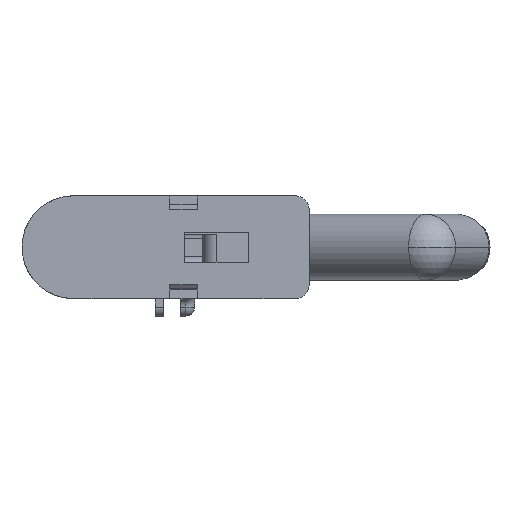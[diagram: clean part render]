
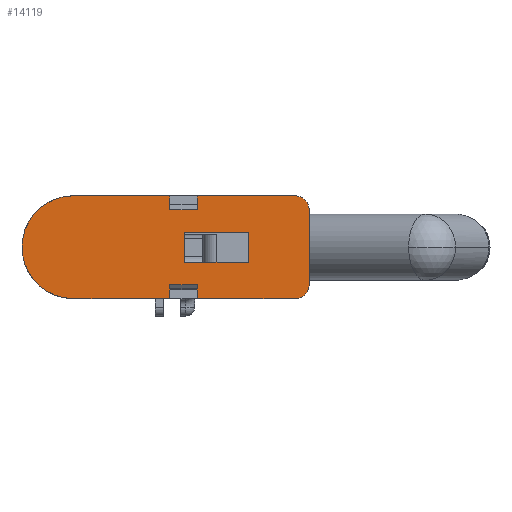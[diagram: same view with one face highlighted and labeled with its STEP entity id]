
A CAD part, left-side view. The second image highlights one B-rep face of the part: STEP entity #14119.
In plain terms, the highlighted planar face has unit normal (-1, 0, 0).
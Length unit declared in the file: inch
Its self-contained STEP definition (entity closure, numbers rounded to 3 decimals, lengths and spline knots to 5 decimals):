
#7 = EDGE_CURVE ( 'NONE', #6480, #2978, #19024, .T. ) ;
#82 = EDGE_CURVE ( 'NONE', #23408, #14286, #2425, .T. ) ;
#172 = DIRECTION ( 'NONE',  ( 0., -1., 0. ) ) ;
#319 = CARTESIAN_POINT ( 'NONE',  ( -5.00064, -0.77841, -0.73097 ) ) ;
#370 = DIRECTION ( 'NONE',  ( -1., 0., 0. ) ) ;
#374 = CARTESIAN_POINT ( 'NONE',  ( -5.00064, -1.89702, 0.21654 ) ) ;
#472 = VERTEX_POINT ( 'NONE', #2930 ) ;
#625 = EDGE_CURVE ( 'NONE', #23710, #17356, #10900, .T. ) ;
#834 = CARTESIAN_POINT ( 'NONE',  ( -5.00064, -0.47716, -0.73097 ) ) ;
#877 = CARTESIAN_POINT ( 'NONE',  ( -5.00064, -2.76317, -0.73097 ) ) ;
#1217 = DIRECTION ( 'NONE',  ( 0., -1., 0. ) ) ;
#1369 = CARTESIAN_POINT ( 'NONE',  ( -5.00064, -1.17211, 0.53412 ) ) ;
#1397 = AXIS2_PLACEMENT_3D ( 'NONE', #12386, #370, #14398 ) ;
#2003 = VECTOR ( 'NONE', #4301, 39.37008 ) ;
#2425 = LINE ( 'NONE', #16116, #3072 ) ;
#2536 = CARTESIAN_POINT ( 'NONE',  ( -5.00064, 0.59382, 0. ) ) ;
#2633 = PLANE ( 'NONE',  #14245 ) ;
#2685 = EDGE_CURVE ( 'NONE', #14286, #5938, #12403, .T. ) ;
#2930 = CARTESIAN_POINT ( 'NONE',  ( -5.00064, -0.77841, -0.53412 ) ) ;
#2978 = VERTEX_POINT ( 'NONE', #20927 ) ;
#3072 = VECTOR ( 'NONE', #172, 39.37008 ) ;
#3211 = ORIENTED_EDGE ( 'NONE', *, *, #15143, .F. ) ;
#3433 = VECTOR ( 'NONE', #15560, 39.37008 ) ;
#3440 = VECTOR ( 'NONE', #15381, 39.37008 ) ;
#3620 = CARTESIAN_POINT ( 'NONE',  ( -5.00064, 0.6158, -0.73097 ) ) ;
#3667 = VECTOR ( 'NONE', #13679, 39.37008 ) ;
#3846 = LINE ( 'NONE', #23876, #19196 ) ;
#3899 = VECTOR ( 'NONE', #14204, 39.37008 ) ;
#4105 = VERTEX_POINT ( 'NONE', #319 ) ;
#4142 = CARTESIAN_POINT ( 'NONE',  ( -5.00064, -0.77841, 0.73097 ) ) ;
#4150 = LINE ( 'NONE', #7176, #24799 ) ;
#4214 = ORIENTED_EDGE ( 'NONE', *, *, #7452, .F. ) ;
#4301 = DIRECTION ( 'NONE',  ( 0., 0., 1. ) ) ;
#4498 = ORIENTED_EDGE ( 'NONE', *, *, #82, .F. ) ;
#4556 = DIRECTION ( 'NONE',  ( 0., 0., 1. ) ) ;
#4612 = ORIENTED_EDGE ( 'NONE', *, *, #17510, .F. ) ;
#4621 = CARTESIAN_POINT ( 'NONE',  ( -5.00064, 0.6158, 0.73097 ) ) ;
#5158 = LINE ( 'NONE', #19234, #25776 ) ;
#5443 = CARTESIAN_POINT ( 'NONE',  ( -5.00064, -1.89702, -0.21654 ) ) ;
#5496 = CARTESIAN_POINT ( 'NONE',  ( -5.00064, -0.77841, -0.73097 ) ) ;
#5601 = AXIS2_PLACEMENT_3D ( 'NONE', #2536, #16521, #4556 ) ;
#5738 = ORIENTED_EDGE ( 'NONE', *, *, #7, .F. ) ;
#5938 = VERTEX_POINT ( 'NONE', #374 ) ;
#6448 = ORIENTED_EDGE ( 'NONE', *, *, #7729, .F. ) ;
#6480 = VERTEX_POINT ( 'NONE', #14417 ) ;
#6512 = DIRECTION ( 'NONE',  ( 0., -1., 0. ) ) ;
#6532 = VECTOR ( 'NONE', #23488, 39.37008 ) ;
#6745 = CARTESIAN_POINT ( 'NONE',  ( -5.00064, 2.30886, -16.99949 ) ) ;
#6814 = EDGE_CURVE ( 'NONE', #11249, #6480, #18746, .T. ) ;
#7101 = VECTOR ( 'NONE', #22167, 39.37008 ) ;
#7171 = CARTESIAN_POINT ( 'NONE',  ( -5.00064, -2.56632, 0.53412 ) ) ;
#7176 = CARTESIAN_POINT ( 'NONE',  ( -5.00064, -0.47716, 0.73097 ) ) ;
#7179 = LINE ( 'NONE', #5496, #6532 ) ;
#7230 = CARTESIAN_POINT ( 'NONE',  ( -5.00064, -0.99151, 0.21654 ) ) ;
#7359 = LINE ( 'NONE', #12258, #2003 ) ;
#7452 = EDGE_CURVE ( 'NONE', #18812, #13443, #23778, .T. ) ;
#7729 = EDGE_CURVE ( 'NONE', #2978, #19135, #8129, .T. ) ;
#7967 = CIRCLE ( 'NONE', #1397, 0.19685 ) ;
#8129 = LINE ( 'NONE', #1369, #3440 ) ;
#8660 = ORIENTED_EDGE ( 'NONE', *, *, #18913, .F. ) ;
#9104 = EDGE_LOOP ( 'NONE', ( #6448, #5738, #21211, #20274, #4214, #25468, #23220, #15988, #4612, #10188, #17609, #23754, #13958, #8660 ) ) ;
#9213 = DIRECTION ( 'NONE',  ( 0., 0., 1. ) ) ;
#9797 = CARTESIAN_POINT ( 'NONE',  ( -5.00064, -0.77841, 0.73097 ) ) ;
#9852 = CARTESIAN_POINT ( 'NONE',  ( -5.00064, -0.77841, 0.53412 ) ) ;
#10070 = VECTOR ( 'NONE', #6512, 39.37008 ) ;
#10188 = ORIENTED_EDGE ( 'NONE', *, *, #15830, .T. ) ;
#10584 = CARTESIAN_POINT ( 'NONE',  ( -5.00064, -1.17211, -0.73097 ) ) ;
#10761 = VERTEX_POINT ( 'NONE', #7230 ) ;
#10817 = EDGE_LOOP ( 'NONE', ( #3211, #17130, #4498, #11124 ) ) ;
#10900 = CIRCLE ( 'NONE', #15709, 0.19685 ) ;
#11124 = ORIENTED_EDGE ( 'NONE', *, *, #17986, .T. ) ;
#11249 = VERTEX_POINT ( 'NONE', #4142 ) ;
#11300 = CARTESIAN_POINT ( 'NONE',  ( -5.00064, -2.76317, 0.53412 ) ) ;
#12134 = EDGE_CURVE ( 'NONE', #14852, #472, #13526, .T. ) ;
#12141 = FACE_OUTER_BOUND ( 'NONE', #9104, .T. ) ;
#12258 = CARTESIAN_POINT ( 'NONE',  ( -5.00064, -1.17211, -0.73097 ) ) ;
#12386 = CARTESIAN_POINT ( 'NONE',  ( -5.00064, -2.56632, -0.53412 ) ) ;
#12403 = LINE ( 'NONE', #24191, #7101 ) ;
#12825 = DIRECTION ( 'NONE',  ( 0., -1., 0. ) ) ;
#13294 = DIRECTION ( 'NONE',  ( 0., 0., 1. ) ) ;
#13336 = DIRECTION ( 'NONE',  ( 0., 1., 0. ) ) ;
#13443 = VERTEX_POINT ( 'NONE', #4621 ) ;
#13526 = LINE ( 'NONE', #25294, #23520 ) ;
#13679 = DIRECTION ( 'NONE',  ( 0., 1., 0. ) ) ;
#13720 = VECTOR ( 'NONE', #21796, 39.37008 ) ;
#13932 = DIRECTION ( 'NONE',  ( 0., -1., 0. ) ) ;
#13958 = ORIENTED_EDGE ( 'NONE', *, *, #625, .T. ) ;
#14119 = ADVANCED_FACE ( 'NONE', ( #12141, #17473 ), #2633, .T. ) ;
#14204 = DIRECTION ( 'NONE',  ( 0., 0., 1. ) ) ;
#14245 = AXIS2_PLACEMENT_3D ( 'NONE', #6745, #16624, #22737 ) ;
#14286 = VERTEX_POINT ( 'NONE', #5443 ) ;
#14312 = LINE ( 'NONE', #23639, #3667 ) ;
#14398 = DIRECTION ( 'NONE',  ( 0., 0., 1. ) ) ;
#14417 = CARTESIAN_POINT ( 'NONE',  ( -5.00064, -0.77841, 0.53412 ) ) ;
#14553 = LINE ( 'NONE', #877, #3899 ) ;
#14852 = VERTEX_POINT ( 'NONE', #24321 ) ;
#15143 = EDGE_CURVE ( 'NONE', #5938, #10761, #14312, .T. ) ;
#15381 = DIRECTION ( 'NONE',  ( 0., 0., 1. ) ) ;
#15401 = LINE ( 'NONE', #20504, #10070 ) ;
#15560 = DIRECTION ( 'NONE',  ( 0., 0., -1. ) ) ;
#15709 = AXIS2_PLACEMENT_3D ( 'NONE', #7171, #21174, #9213 ) ;
#15830 = EDGE_CURVE ( 'NONE', #16779, #16683, #23048, .T. ) ;
#15988 = ORIENTED_EDGE ( 'NONE', *, *, #12134, .F. ) ;
#16116 = CARTESIAN_POINT ( 'NONE',  ( -5.00064, 0., -0.21654 ) ) ;
#16521 = DIRECTION ( 'NONE',  ( 1., 0., 0. ) ) ;
#16623 = CARTESIAN_POINT ( 'NONE',  ( -5.00064, -2.76317, -0.53412 ) ) ;
#16624 = DIRECTION ( 'NONE',  ( -1., 0., 0. ) ) ;
#16683 = VERTEX_POINT ( 'NONE', #18884 ) ;
#16779 = VERTEX_POINT ( 'NONE', #10584 ) ;
#17130 = ORIENTED_EDGE ( 'NONE', *, *, #2685, .F. ) ;
#17356 = VERTEX_POINT ( 'NONE', #19100 ) ;
#17473 = FACE_BOUND ( 'NONE', #10817, .T. ) ;
#17510 = EDGE_CURVE ( 'NONE', #16779, #14852, #7359, .T. ) ;
#17609 = ORIENTED_EDGE ( 'NONE', *, *, #18152, .T. ) ;
#17986 = EDGE_CURVE ( 'NONE', #23408, #10761, #5158, .T. ) ;
#18152 = EDGE_CURVE ( 'NONE', #16683, #19073, #7967, .T. ) ;
#18746 = LINE ( 'NONE', #9797, #3433 ) ;
#18812 = VERTEX_POINT ( 'NONE', #3620 ) ;
#18884 = CARTESIAN_POINT ( 'NONE',  ( -5.00064, -2.56632, -0.73097 ) ) ;
#18913 = EDGE_CURVE ( 'NONE', #19135, #17356, #3846, .T. ) ;
#19024 = LINE ( 'NONE', #9852, #13720 ) ;
#19073 = VERTEX_POINT ( 'NONE', #16623 ) ;
#19100 = CARTESIAN_POINT ( 'NONE',  ( -5.00064, -2.56632, 0.73097 ) ) ;
#19135 = VERTEX_POINT ( 'NONE', #22823 ) ;
#19196 = VECTOR ( 'NONE', #13932, 39.37008 ) ;
#19199 = EDGE_CURVE ( 'NONE', #13443, #11249, #4150, .T. ) ;
#19234 = CARTESIAN_POINT ( 'NONE',  ( -5.00064, -0.99151, 0. ) ) ;
#20203 = CARTESIAN_POINT ( 'NONE',  ( -5.00064, -0.99151, -0.21654 ) ) ;
#20274 = ORIENTED_EDGE ( 'NONE', *, *, #19199, .F. ) ;
#20504 = CARTESIAN_POINT ( 'NONE',  ( -5.00064, -0.47716, -0.73097 ) ) ;
#20927 = CARTESIAN_POINT ( 'NONE',  ( -5.00064, -1.17211, 0.53412 ) ) ;
#21174 = DIRECTION ( 'NONE',  ( -1., 0., 0. ) ) ;
#21211 = ORIENTED_EDGE ( 'NONE', *, *, #6814, .F. ) ;
#21796 = DIRECTION ( 'NONE',  ( 0., -1., 0. ) ) ;
#22167 = DIRECTION ( 'NONE',  ( 0., 0., 1. ) ) ;
#22295 = EDGE_CURVE ( 'NONE', #472, #4105, #7179, .T. ) ;
#22374 = VECTOR ( 'NONE', #12825, 39.37008 ) ;
#22737 = DIRECTION ( 'NONE',  ( 0., 0., 1. ) ) ;
#22823 = CARTESIAN_POINT ( 'NONE',  ( -5.00064, -1.17211, 0.73097 ) ) ;
#22897 = EDGE_CURVE ( 'NONE', #19073, #23710, #14553, .T. ) ;
#23048 = LINE ( 'NONE', #834, #22374 ) ;
#23220 = ORIENTED_EDGE ( 'NONE', *, *, #22295, .F. ) ;
#23408 = VERTEX_POINT ( 'NONE', #20203 ) ;
#23488 = DIRECTION ( 'NONE',  ( 0., 0., -1. ) ) ;
#23520 = VECTOR ( 'NONE', #13336, 39.37008 ) ;
#23639 = CARTESIAN_POINT ( 'NONE',  ( -5.00064, 0., 0.21654 ) ) ;
#23710 = VERTEX_POINT ( 'NONE', #11300 ) ;
#23754 = ORIENTED_EDGE ( 'NONE', *, *, #22897, .T. ) ;
#23778 = CIRCLE ( 'NONE', #5601, 0.7313 ) ;
#23876 = CARTESIAN_POINT ( 'NONE',  ( -5.00064, -0.47716, 0.73097 ) ) ;
#24191 = CARTESIAN_POINT ( 'NONE',  ( -5.00064, -1.89702, -0.21654 ) ) ;
#24321 = CARTESIAN_POINT ( 'NONE',  ( -5.00064, -1.17211, -0.53412 ) ) ;
#24799 = VECTOR ( 'NONE', #1217, 39.37008 ) ;
#25294 = CARTESIAN_POINT ( 'NONE',  ( -5.00064, -1.17211, -0.53412 ) ) ;
#25468 = ORIENTED_EDGE ( 'NONE', *, *, #25727, .T. ) ;
#25727 = EDGE_CURVE ( 'NONE', #18812, #4105, #15401, .T. ) ;
#25776 = VECTOR ( 'NONE', #13294, 39.37008 ) ;
